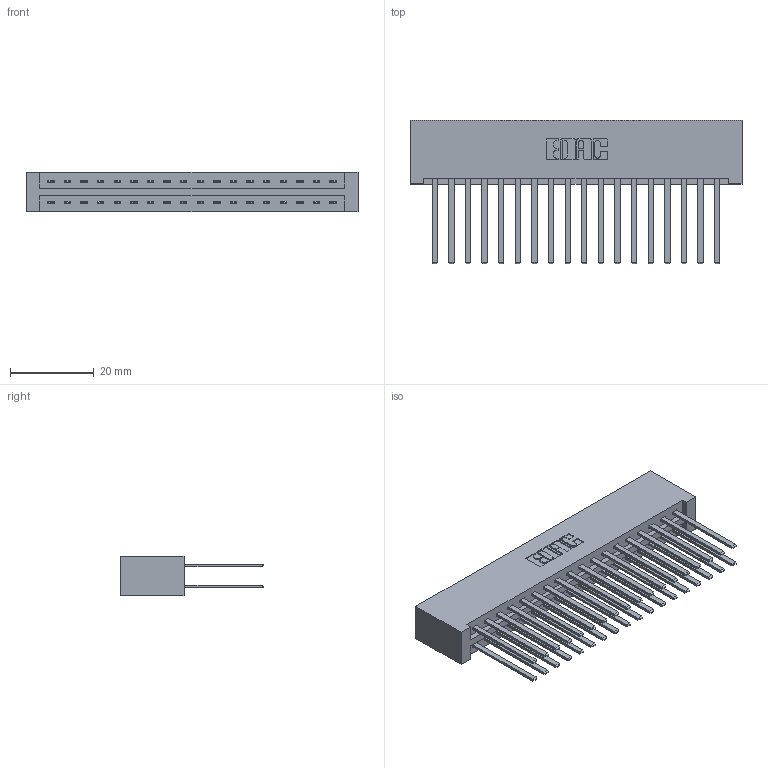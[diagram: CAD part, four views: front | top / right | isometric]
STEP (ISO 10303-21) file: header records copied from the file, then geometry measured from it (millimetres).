
FILE_DESCRIPTION (( 'STEP AP203' ), '1' );
FILE_NAME ('337-036-544-201.STEP', '2019-10-08T20:59:23', ( '' ), ( '' ), 'SwSTEP 2.0', 'SolidWorks 2016', '' );
FILE_SCHEMA (( 'CONFIG_CONTROL_DESIGN' ));
Length unit declared in the file: inch
Products named in the file (3): 345-292-001_345-293-144; 337-036-544-201; 337 Part_No Mounting Lugs
Assembly tree (37 placements, depth 2):
  337-036-544-201
    337 Part_No Mounting Lugs
    345-292-001_345-293-144  x36
Bounding box: 79.2 x 34.3 x 9.4 mm (x, y, z)
Volume: 9292.4 mm3; surface area: 11976.6 mm2
Topology: 37 solids, 37 shells, 1834 faces, 5435 edges, 3574 vertices
Faces by surface type: plane 1290, cylinder 544
Entity records: 16599 total; most frequent: CARTESIAN_POINT 2814, ORIENTED_EDGE 2750, DIRECTION 2427, EDGE_CURVE 1375, LINE 1259, VECTOR 1259, VERTEX_POINT 914, AXIS2_PLACEMENT_3D 584
